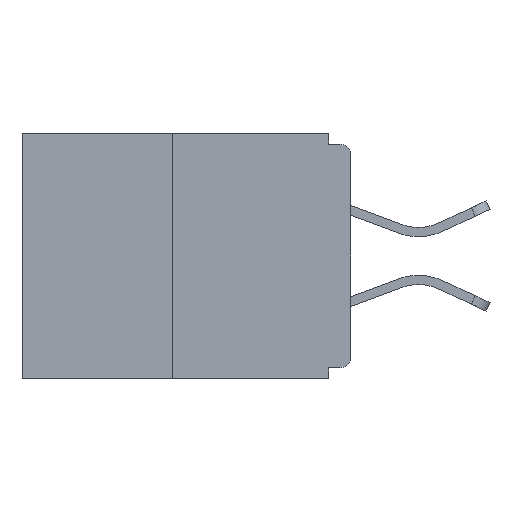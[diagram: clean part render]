
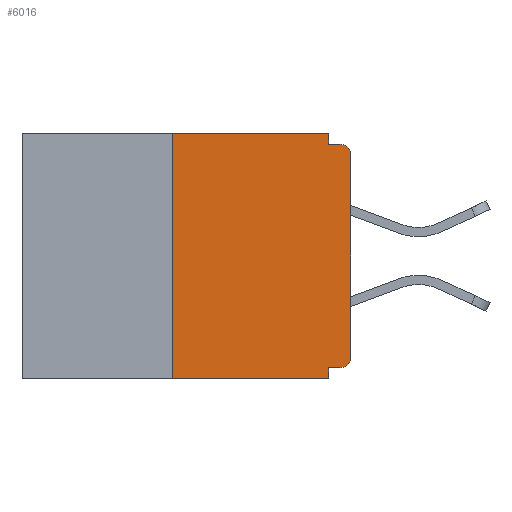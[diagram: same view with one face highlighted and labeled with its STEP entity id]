
A CAD part, left-side view. The second image highlights one B-rep face of the part: STEP entity #6016.
In plain terms, the highlighted planar face has unit normal (-1, 0, 0).
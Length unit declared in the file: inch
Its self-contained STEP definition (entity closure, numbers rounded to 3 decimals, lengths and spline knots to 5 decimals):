
#215 = VERTEX_POINT ( 'NONE', #1392 ) ;
#488 = EDGE_CURVE ( 'NONE', #6911, #5135, #6158, .T. ) ;
#530 = PLANE ( 'NONE',  #1146 ) ;
#578 = CARTESIAN_POINT ( 'NONE',  ( 0., 0.031, -0.343 ) ) ;
#721 = DIRECTION ( 'NONE',  ( 0., 1., 0. ) ) ;
#841 = CARTESIAN_POINT ( 'NONE',  ( 0., 0.031, 0. ) ) ;
#1013 = DIRECTION ( 'NONE',  ( -1., 0., 0. ) ) ;
#1146 = AXIS2_PLACEMENT_3D ( 'NONE', #3531, #2643, #1621 ) ;
#1361 = DIRECTION ( 'NONE',  ( 0., -1., 0. ) ) ;
#1370 = ORIENTED_EDGE ( 'NONE', *, *, #2072, .F. ) ;
#1392 = CARTESIAN_POINT ( 'NONE',  ( 0., 0., -0.03 ) ) ;
#1473 = LINE ( 'NONE', #3648, #3853 ) ;
#1621 = DIRECTION ( 'NONE',  ( 0., 0., -1. ) ) ;
#1692 = CARTESIAN_POINT ( 'NONE',  ( 0., 0.46, -0.343 ) ) ;
#1723 = AXIS2_PLACEMENT_3D ( 'NONE', #2688, #2886, #8875 ) ;
#1893 = CARTESIAN_POINT ( 'NONE',  ( 0., 0.46, 0. ) ) ;
#2072 = EDGE_CURVE ( 'NONE', #3573, #6911, #1473, .T. ) ;
#2249 = DIRECTION ( 'NONE',  ( 0., 0., 1. ) ) ;
#2306 = DIRECTION ( 'NONE',  ( 0., 0., -1. ) ) ;
#2643 = DIRECTION ( 'NONE',  ( 1., 0., 0. ) ) ;
#2688 = CARTESIAN_POINT ( 'NONE',  ( 0., 0.015, -0.313 ) ) ;
#2886 = DIRECTION ( 'NONE',  ( -1., 0., 0. ) ) ;
#2945 = CARTESIAN_POINT ( 'NONE',  ( 0., 0.015, -0.328 ) ) ;
#3046 = CARTESIAN_POINT ( 'NONE',  ( 0., 0.25, 0. ) ) ;
#3531 = CARTESIAN_POINT ( 'NONE',  ( 0., 0.46, 0. ) ) ;
#3573 = VERTEX_POINT ( 'NONE', #2945 ) ;
#3648 = CARTESIAN_POINT ( 'NONE',  ( 0., 0., -0.328 ) ) ;
#3770 = VERTEX_POINT ( 'NONE', #4369 ) ;
#3853 = VECTOR ( 'NONE', #721, 39.37008 ) ;
#3997 = ORIENTED_EDGE ( 'NONE', *, *, #4867, .F. ) ;
#4354 = CARTESIAN_POINT ( 'NONE',  ( 0., 0.015, -0.015 ) ) ;
#4369 = CARTESIAN_POINT ( 'NONE',  ( 0., 0.25, 0. ) ) ;
#4608 = EDGE_CURVE ( 'NONE', #11025, #215, #5360, .T. ) ;
#4625 = VECTOR ( 'NONE', #11011, 39.37008 ) ;
#4692 = LINE ( 'NONE', #9664, #12168 ) ;
#4867 = EDGE_CURVE ( 'NONE', #11892, #8599, #11341, .T. ) ;
#4952 = EDGE_CURVE ( 'NONE', #11740, #3770, #7979, .T. ) ;
#5135 = VERTEX_POINT ( 'NONE', #578 ) ;
#5360 = LINE ( 'NONE', #11488, #10829 ) ;
#5361 = ORIENTED_EDGE ( 'NONE', *, *, #4952, .F. ) ;
#5507 = EDGE_LOOP ( 'NONE', ( #7181, #5361, #12335, #12604, #1370, #10842, #7553, #12265, #5919, #3997 ) ) ;
#5910 = LINE ( 'NONE', #1893, #4625 ) ;
#5919 = ORIENTED_EDGE ( 'NONE', *, *, #7253, .F. ) ;
#5972 = LINE ( 'NONE', #1692, #6571 ) ;
#6016 = ADVANCED_FACE ( 'NONE', ( #10942 ), #530, .F. ) ;
#6158 = LINE ( 'NONE', #7174, #10077 ) ;
#6571 = VECTOR ( 'NONE', #13271, 39.37008 ) ;
#6885 = CARTESIAN_POINT ( 'NONE',  ( 0., 0.031, -0.328 ) ) ;
#6911 = VERTEX_POINT ( 'NONE', #6885 ) ;
#7141 = CARTESIAN_POINT ( 'NONE',  ( 0., 0.031, -0.015 ) ) ;
#7174 = CARTESIAN_POINT ( 'NONE',  ( 0., 0.031, -0.343 ) ) ;
#7181 = ORIENTED_EDGE ( 'NONE', *, *, #10417, .F. ) ;
#7253 = EDGE_CURVE ( 'NONE', #8599, #10117, #4692, .T. ) ;
#7553 = ORIENTED_EDGE ( 'NONE', *, *, #4608, .T. ) ;
#7645 = VECTOR ( 'NONE', #13392, 39.37008 ) ;
#7979 = LINE ( 'NONE', #3046, #10678 ) ;
#8186 = EDGE_CURVE ( 'NONE', #3573, #11025, #10418, .T. ) ;
#8599 = VERTEX_POINT ( 'NONE', #7141 ) ;
#8758 = EDGE_CURVE ( 'NONE', #215, #10117, #10429, .T. ) ;
#8875 = DIRECTION ( 'NONE',  ( 0., 0., -1. ) ) ;
#9216 = DIRECTION ( 'NONE',  ( 0., 0., -1. ) ) ;
#9664 = CARTESIAN_POINT ( 'NONE',  ( 0., 0., -0.015 ) ) ;
#10077 = VECTOR ( 'NONE', #9216, 39.37008 ) ;
#10117 = VERTEX_POINT ( 'NONE', #4354 ) ;
#10379 = CARTESIAN_POINT ( 'NONE',  ( 0., 0., -0.313 ) ) ;
#10417 = EDGE_CURVE ( 'NONE', #3770, #11892, #5910, .T. ) ;
#10418 = CIRCLE ( 'NONE', #1723, 0.015 ) ;
#10429 = CIRCLE ( 'NONE', #12824, 0.015 ) ;
#10433 = EDGE_CURVE ( 'NONE', #11740, #5135, #5972, .T. ) ;
#10678 = VECTOR ( 'NONE', #13260, 39.37008 ) ;
#10829 = VECTOR ( 'NONE', #2249, 39.37008 ) ;
#10842 = ORIENTED_EDGE ( 'NONE', *, *, #8186, .T. ) ;
#10942 = FACE_OUTER_BOUND ( 'NONE', #5507, .T. ) ;
#10976 = CARTESIAN_POINT ( 'NONE',  ( 0., 0.25, -0.343 ) ) ;
#11011 = DIRECTION ( 'NONE',  ( 0., -1., 0. ) ) ;
#11025 = VERTEX_POINT ( 'NONE', #10379 ) ;
#11341 = LINE ( 'NONE', #12160, #7645 ) ;
#11488 = CARTESIAN_POINT ( 'NONE',  ( 0., 0., 0. ) ) ;
#11740 = VERTEX_POINT ( 'NONE', #10976 ) ;
#11892 = VERTEX_POINT ( 'NONE', #841 ) ;
#12160 = CARTESIAN_POINT ( 'NONE',  ( 0., 0.031, 0. ) ) ;
#12168 = VECTOR ( 'NONE', #1361, 39.37008 ) ;
#12265 = ORIENTED_EDGE ( 'NONE', *, *, #8758, .T. ) ;
#12335 = ORIENTED_EDGE ( 'NONE', *, *, #10433, .T. ) ;
#12604 = ORIENTED_EDGE ( 'NONE', *, *, #488, .F. ) ;
#12824 = AXIS2_PLACEMENT_3D ( 'NONE', #13275, #1013, #2306 ) ;
#13260 = DIRECTION ( 'NONE',  ( 0., 0., 1. ) ) ;
#13271 = DIRECTION ( 'NONE',  ( 0., -1., 0. ) ) ;
#13275 = CARTESIAN_POINT ( 'NONE',  ( 0., 0.015, -0.03 ) ) ;
#13392 = DIRECTION ( 'NONE',  ( 0., 0., -1. ) ) ;
